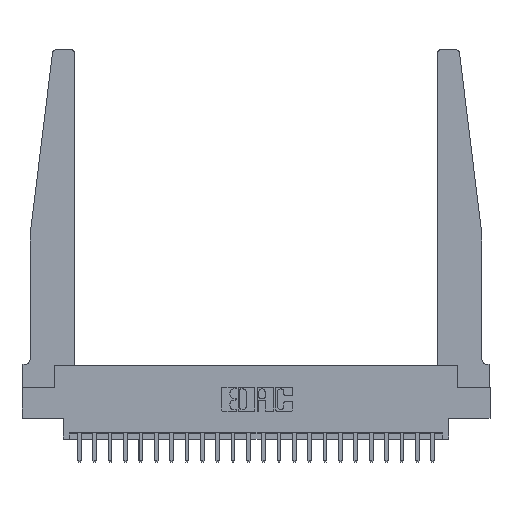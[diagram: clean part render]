
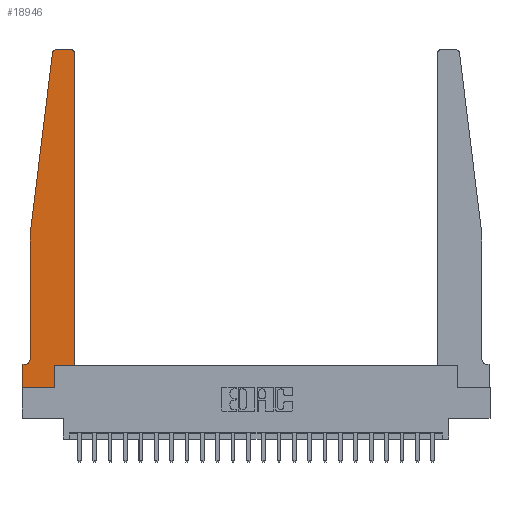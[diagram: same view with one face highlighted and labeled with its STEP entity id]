
A CAD part, top view. The second image highlights one B-rep face of the part: STEP entity #18946.
In plain terms, the highlighted planar face has unit normal (0, 0, 1).
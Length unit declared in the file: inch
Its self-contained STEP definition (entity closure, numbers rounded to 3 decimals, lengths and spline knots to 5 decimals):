
#25 = DIRECTION ( 'NONE',  ( 0., 0., 1. ) ) ;
#53 = DIRECTION ( 'NONE',  ( -1., 0., 0. ) ) ;
#540 = CARTESIAN_POINT ( 'NONE',  ( 0.425, 0.18, 0.37 ) ) ;
#753 = CARTESIAN_POINT ( 'NONE',  ( 0.015, 0.1875, 0.37 ) ) ;
#819 = EDGE_CURVE ( 'NONE', #6622, #5608, #4318, .T. ) ;
#1007 = EDGE_CURVE ( 'NONE', #17906, #6451, #5753, .T. ) ;
#1334 = VECTOR ( 'NONE', #20489, 39.37008 ) ;
#2015 = CARTESIAN_POINT ( 'NONE',  ( 0.25, 2.75, 0.37 ) ) ;
#2421 = VECTOR ( 'NONE', #17791, 39.37008 ) ;
#2989 = CARTESIAN_POINT ( 'NONE',  ( 0.425, 2.72, 0.37 ) ) ;
#3588 = CARTESIAN_POINT ( 'NONE',  ( 0., 0.1875, 0.37 ) ) ;
#3701 = EDGE_CURVE ( 'NONE', #18491, #12620, #4792, .T. ) ;
#3813 = DIRECTION ( 'NONE',  ( 0., 0., -1. ) ) ;
#4130 = CARTESIAN_POINT ( 'NONE',  ( 0.065, 1.25, 0.37 ) ) ;
#4290 = CARTESIAN_POINT ( 'NONE',  ( 0.2605, 0.18, 0.37 ) ) ;
#4318 = CIRCLE ( 'NONE', #5190, 0.03 ) ;
#4533 = LINE ( 'NONE', #11083, #19147 ) ;
#4662 = VERTEX_POINT ( 'NONE', #10410 ) ;
#4784 = VECTOR ( 'NONE', #20132, 39.37008 ) ;
#4792 = LINE ( 'NONE', #540, #18871 ) ;
#5190 = AXIS2_PLACEMENT_3D ( 'NONE', #11240, #9711, #7068 ) ;
#5272 = LINE ( 'NONE', #4290, #14765 ) ;
#5464 = DIRECTION ( 'NONE',  ( 1., 0., 0. ) ) ;
#5608 = VERTEX_POINT ( 'NONE', #11062 ) ;
#5753 = LINE ( 'NONE', #19499, #1334 ) ;
#6309 = EDGE_CURVE ( 'NONE', #4662, #19284, #12337, .T. ) ;
#6440 = VERTEX_POINT ( 'NONE', #4130 ) ;
#6451 = VERTEX_POINT ( 'NONE', #14854 ) ;
#6622 = VERTEX_POINT ( 'NONE', #15273 ) ;
#7068 = DIRECTION ( 'NONE',  ( 1., 0., 0. ) ) ;
#7120 = AXIS2_PLACEMENT_3D ( 'NONE', #3588, #16071, #5464 ) ;
#7141 = CARTESIAN_POINT ( 'NONE',  ( 0.065, 1.25, 0.37 ) ) ;
#7605 = LINE ( 'NONE', #14601, #12345 ) ;
#7933 = DIRECTION ( 'NONE',  ( 0., 1., 0. ) ) ;
#8154 = EDGE_CURVE ( 'NONE', #9600, #21020, #5272, .T. ) ;
#8263 = VECTOR ( 'NONE', #21153, 39.37008 ) ;
#9163 = VERTEX_POINT ( 'NONE', #20860 ) ;
#9600 = VERTEX_POINT ( 'NONE', #15257 ) ;
#9711 = DIRECTION ( 'NONE',  ( 0., 0., 1. ) ) ;
#9953 = EDGE_CURVE ( 'NONE', #12620, #9163, #20596, .T. ) ;
#10410 = CARTESIAN_POINT ( 'NONE',  ( 0.065, 0.2375, 0.37 ) ) ;
#10887 = AXIS2_PLACEMENT_3D ( 'NONE', #14548, #3813, #16264 ) ;
#11052 = CARTESIAN_POINT ( 'NONE',  ( 0.395, 2.72, 0.37 ) ) ;
#11062 = CARTESIAN_POINT ( 'NONE',  ( 0.24675, 2.72367, 0.37 ) ) ;
#11083 = CARTESIAN_POINT ( 'NONE',  ( 0.425, 0.18, 0.37 ) ) ;
#11240 = CARTESIAN_POINT ( 'NONE',  ( 0.27653, 2.72, 0.37 ) ) ;
#11333 = CARTESIAN_POINT ( 'NONE',  ( 0., 0.1875, 0.37 ) ) ;
#11668 = CARTESIAN_POINT ( 'NONE',  ( 0.2605, 0.18, 0.37 ) ) ;
#11766 = EDGE_CURVE ( 'NONE', #6440, #4662, #13522, .T. ) ;
#12060 = LINE ( 'NONE', #12626, #2421 ) ;
#12337 = CIRCLE ( 'NONE', #10887, 0.05 ) ;
#12345 = VECTOR ( 'NONE', #53, 39.37008 ) ;
#12420 = EDGE_CURVE ( 'NONE', #6451, #9600, #18867, .T. ) ;
#12434 = PLANE ( 'NONE',  #7120 ) ;
#12620 = VERTEX_POINT ( 'NONE', #2989 ) ;
#12626 = CARTESIAN_POINT ( 'NONE',  ( 0.065, 1.25, 0.37 ) ) ;
#12820 = DIRECTION ( 'NONE',  ( 1., 0., 0. ) ) ;
#13516 = EDGE_CURVE ( 'NONE', #5608, #6440, #12060, .T. ) ;
#13522 = LINE ( 'NONE', #7141, #8263 ) ;
#13635 = EDGE_LOOP ( 'NONE', ( #18584, #20777, #22250, #18155, #20559, #20517, #21369, #22450, #20205, #17821, #18955, #18469 ) ) ;
#14526 = DIRECTION ( 'NONE',  ( 1., 0., 0. ) ) ;
#14548 = CARTESIAN_POINT ( 'NONE',  ( 0.015, 0.2375, 0.37 ) ) ;
#14601 = CARTESIAN_POINT ( 'NONE',  ( 0.065, 0.1875, 0.37 ) ) ;
#14765 = VECTOR ( 'NONE', #16698, 39.37008 ) ;
#14789 = FACE_OUTER_BOUND ( 'NONE', #13635, .T. ) ;
#14854 = CARTESIAN_POINT ( 'NONE',  ( 0., 0., 0.37 ) ) ;
#15257 = CARTESIAN_POINT ( 'NONE',  ( 0.2605, 0., 0.37 ) ) ;
#15273 = CARTESIAN_POINT ( 'NONE',  ( 0.27653, 2.75, 0.37 ) ) ;
#16071 = DIRECTION ( 'NONE',  ( 0., 0., 1. ) ) ;
#16264 = DIRECTION ( 'NONE',  ( -1., 0., 0. ) ) ;
#16365 = DIRECTION ( 'NONE',  ( -1., 0., 0. ) ) ;
#16698 = DIRECTION ( 'NONE',  ( 0., 1., 0. ) ) ;
#17308 = LINE ( 'NONE', #2015, #22520 ) ;
#17791 = DIRECTION ( 'NONE',  ( -0.122, -0.992, 0. ) ) ;
#17821 = ORIENTED_EDGE ( 'NONE', *, *, #22648, .T. ) ;
#17906 = VERTEX_POINT ( 'NONE', #11333 ) ;
#18155 = ORIENTED_EDGE ( 'NONE', *, *, #11766, .T. ) ;
#18246 = CARTESIAN_POINT ( 'NONE',  ( 0.425, 0.18, 0.37 ) ) ;
#18380 = CARTESIAN_POINT ( 'NONE',  ( 0., 0., 0.37 ) ) ;
#18381 = EDGE_CURVE ( 'NONE', #19284, #17906, #7605, .T. ) ;
#18469 = ORIENTED_EDGE ( 'NONE', *, *, #9953, .T. ) ;
#18491 = VERTEX_POINT ( 'NONE', #18246 ) ;
#18584 = ORIENTED_EDGE ( 'NONE', *, *, #21525, .T. ) ;
#18867 = LINE ( 'NONE', #18380, #4784 ) ;
#18871 = VECTOR ( 'NONE', #7933, 39.37008 ) ;
#18946 = ADVANCED_FACE ( 'NONE', ( #14789 ), #12434, .T. ) ;
#18955 = ORIENTED_EDGE ( 'NONE', *, *, #3701, .T. ) ;
#19147 = VECTOR ( 'NONE', #14526, 39.37008 ) ;
#19284 = VERTEX_POINT ( 'NONE', #753 ) ;
#19499 = CARTESIAN_POINT ( 'NONE',  ( 0., 0., 0.37 ) ) ;
#20132 = DIRECTION ( 'NONE',  ( 1., 0., 0. ) ) ;
#20205 = ORIENTED_EDGE ( 'NONE', *, *, #8154, .T. ) ;
#20483 = AXIS2_PLACEMENT_3D ( 'NONE', #11052, #25, #12820 ) ;
#20489 = DIRECTION ( 'NONE',  ( 0., -1., 0. ) ) ;
#20517 = ORIENTED_EDGE ( 'NONE', *, *, #18381, .T. ) ;
#20559 = ORIENTED_EDGE ( 'NONE', *, *, #6309, .T. ) ;
#20596 = CIRCLE ( 'NONE', #20483, 0.03 ) ;
#20777 = ORIENTED_EDGE ( 'NONE', *, *, #819, .T. ) ;
#20860 = CARTESIAN_POINT ( 'NONE',  ( 0.395, 2.75, 0.37 ) ) ;
#21020 = VERTEX_POINT ( 'NONE', #11668 ) ;
#21153 = DIRECTION ( 'NONE',  ( 0., -1., 0. ) ) ;
#21369 = ORIENTED_EDGE ( 'NONE', *, *, #1007, .T. ) ;
#21525 = EDGE_CURVE ( 'NONE', #9163, #6622, #17308, .T. ) ;
#22250 = ORIENTED_EDGE ( 'NONE', *, *, #13516, .T. ) ;
#22450 = ORIENTED_EDGE ( 'NONE', *, *, #12420, .T. ) ;
#22520 = VECTOR ( 'NONE', #16365, 39.37008 ) ;
#22648 = EDGE_CURVE ( 'NONE', #21020, #18491, #4533, .T. ) ;
